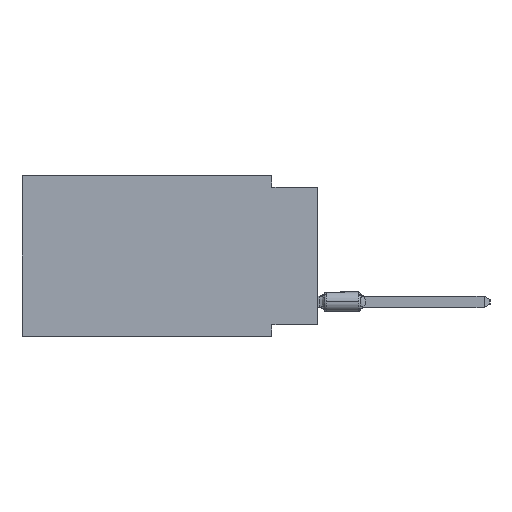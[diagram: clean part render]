
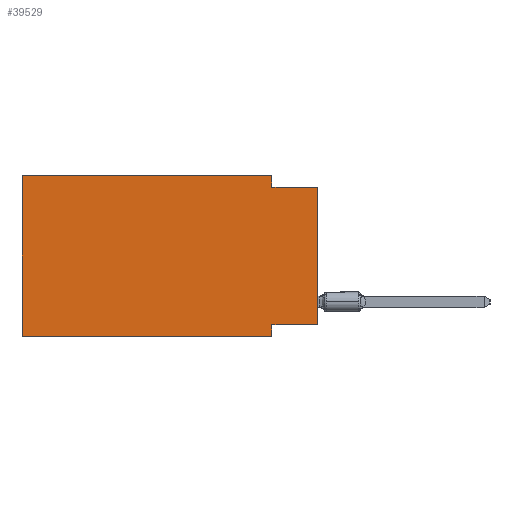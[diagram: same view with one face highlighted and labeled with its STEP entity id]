
A CAD part, left-side view. The second image highlights one B-rep face of the part: STEP entity #39529.
In plain terms, the highlighted planar face has unit normal (-1, 0, 0).
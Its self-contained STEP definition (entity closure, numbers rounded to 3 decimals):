
#282 = VECTOR ( 'NONE', #17415, 1000. ) ;
#370 = LINE ( 'NONE', #914, #282 ) ;
#411 = ORIENTED_EDGE ( 'NONE', *, *, #42008, .T. ) ;
#650 = EDGE_LOOP ( 'NONE', ( #45764, #25217, #41074, #48333, #31756, #411, #45541, #6774 ) ) ;
#780 = EDGE_CURVE ( 'NONE', #33545, #32049, #36781, .T. ) ;
#914 = CARTESIAN_POINT ( 'NONE',  ( 0., 16.383, 0. ) ) ;
#958 = VECTOR ( 'NONE', #39722, 1000. ) ;
#1068 = CARTESIAN_POINT ( 'NONE',  ( 0., 2.54, -8.89 ) ) ;
#2586 = VECTOR ( 'NONE', #4505, 1000. ) ;
#3333 = CARTESIAN_POINT ( 'NONE',  ( 0., 2.54, -8.255 ) ) ;
#4505 = DIRECTION ( 'NONE',  ( 0., -1., 0. ) ) ;
#4646 = CARTESIAN_POINT ( 'NONE',  ( 0., 0., -8.255 ) ) ;
#5858 = FACE_OUTER_BOUND ( 'NONE', #650, .T. ) ;
#6077 = CARTESIAN_POINT ( 'NONE',  ( 0., 2.54, 0. ) ) ;
#6512 = VERTEX_POINT ( 'NONE', #10654 ) ;
#6774 = ORIENTED_EDGE ( 'NONE', *, *, #780, .F. ) ;
#7056 = VERTEX_POINT ( 'NONE', #7790 ) ;
#7790 = CARTESIAN_POINT ( 'NONE',  ( 0., 2.54, -0.635 ) ) ;
#9451 = VECTOR ( 'NONE', #24497, 1000. ) ;
#9733 = DIRECTION ( 'NONE',  ( 0., 0., -1. ) ) ;
#9783 = PLANE ( 'NONE',  #22200 ) ;
#10654 = CARTESIAN_POINT ( 'NONE',  ( 0., 16.383, 0. ) ) ;
#10694 = EDGE_CURVE ( 'NONE', #41206, #6512, #370, .T. ) ;
#15415 = DIRECTION ( 'NONE',  ( 0., -1., 0. ) ) ;
#17415 = DIRECTION ( 'NONE',  ( 0., 0., 1. ) ) ;
#18118 = DIRECTION ( 'NONE',  ( 0., 0., -1. ) ) ;
#21285 = DIRECTION ( 'NONE',  ( 0., 0., 1. ) ) ;
#21878 = EDGE_CURVE ( 'NONE', #33545, #23452, #42242, .T. ) ;
#22095 = VECTOR ( 'NONE', #18118, 1000. ) ;
#22200 = AXIS2_PLACEMENT_3D ( 'NONE', #30741, #22617, #35729 ) ;
#22297 = LINE ( 'NONE', #1068, #22095 ) ;
#22617 = DIRECTION ( 'NONE',  ( 1., 0., 0. ) ) ;
#23379 = EDGE_CURVE ( 'NONE', #6512, #37832, #24070, .T. ) ;
#23452 = VERTEX_POINT ( 'NONE', #46686 ) ;
#24070 = LINE ( 'NONE', #29091, #44157 ) ;
#24497 = DIRECTION ( 'NONE',  ( 0., 1., 0. ) ) ;
#25217 = ORIENTED_EDGE ( 'NONE', *, *, #38206, .F. ) ;
#25312 = VECTOR ( 'NONE', #21285, 1000. ) ;
#26263 = LINE ( 'NONE', #52236, #2586 ) ;
#27354 = CARTESIAN_POINT ( 'NONE',  ( 0., 16.383, -8.89 ) ) ;
#29091 = CARTESIAN_POINT ( 'NONE',  ( 0., 16.383, 0. ) ) ;
#30741 = CARTESIAN_POINT ( 'NONE',  ( 0., 16.383, 0. ) ) ;
#30958 = LINE ( 'NONE', #6077, #39733 ) ;
#31756 = ORIENTED_EDGE ( 'NONE', *, *, #10694, .F. ) ;
#32049 = VERTEX_POINT ( 'NONE', #3333 ) ;
#32073 = VERTEX_POINT ( 'NONE', #46893 ) ;
#33545 = VERTEX_POINT ( 'NONE', #4646 ) ;
#34442 = EDGE_CURVE ( 'NONE', #37832, #7056, #30958, .T. ) ;
#35529 = LINE ( 'NONE', #48637, #958 ) ;
#35729 = DIRECTION ( 'NONE',  ( 0., 0., -1. ) ) ;
#36237 = EDGE_CURVE ( 'NONE', #32049, #32073, #22297, .T. ) ;
#36781 = LINE ( 'NONE', #37341, #9451 ) ;
#37341 = CARTESIAN_POINT ( 'NONE',  ( 0., 0., -8.255 ) ) ;
#37832 = VERTEX_POINT ( 'NONE', #50444 ) ;
#38206 = EDGE_CURVE ( 'NONE', #7056, #23452, #26263, .T. ) ;
#39529 = ADVANCED_FACE ( 'NONE', ( #5858 ), #9783, .F. ) ;
#39722 = DIRECTION ( 'NONE',  ( 0., -1., 0. ) ) ;
#39733 = VECTOR ( 'NONE', #9733, 1000. ) ;
#41074 = ORIENTED_EDGE ( 'NONE', *, *, #34442, .F. ) ;
#41206 = VERTEX_POINT ( 'NONE', #27354 ) ;
#42008 = EDGE_CURVE ( 'NONE', #41206, #32073, #35529, .T. ) ;
#42242 = LINE ( 'NONE', #46431, #25312 ) ;
#44157 = VECTOR ( 'NONE', #15415, 1000. ) ;
#45541 = ORIENTED_EDGE ( 'NONE', *, *, #36237, .F. ) ;
#45764 = ORIENTED_EDGE ( 'NONE', *, *, #21878, .T. ) ;
#46431 = CARTESIAN_POINT ( 'NONE',  ( 0., 0., 0. ) ) ;
#46686 = CARTESIAN_POINT ( 'NONE',  ( 0., 0., -0.635 ) ) ;
#46893 = CARTESIAN_POINT ( 'NONE',  ( 0., 2.54, -8.89 ) ) ;
#48333 = ORIENTED_EDGE ( 'NONE', *, *, #23379, .F. ) ;
#48637 = CARTESIAN_POINT ( 'NONE',  ( 0., 16.383, -8.89 ) ) ;
#50444 = CARTESIAN_POINT ( 'NONE',  ( 0., 2.54, 0. ) ) ;
#52236 = CARTESIAN_POINT ( 'NONE',  ( 0., 0., -0.635 ) ) ;
